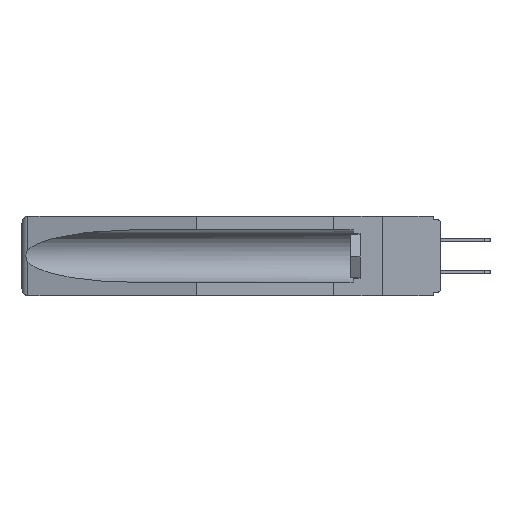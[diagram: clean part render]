
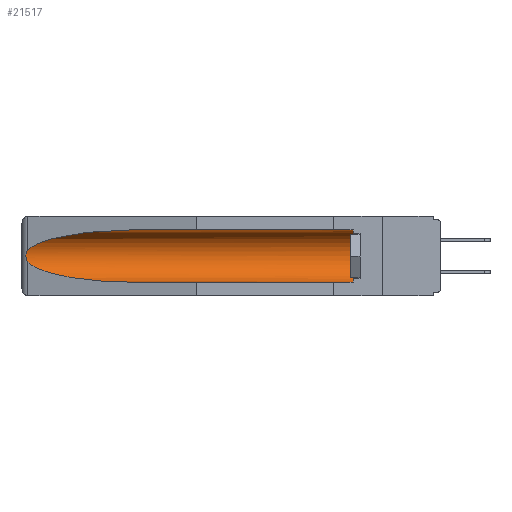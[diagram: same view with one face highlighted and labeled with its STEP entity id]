
A CAD part, left-side view. The second image highlights one B-rep face of the part: STEP entity #21517.
In plain terms, the highlighted cylindrical face has radius 2.857 mm (diameter 5.715 mm), a partial arc.
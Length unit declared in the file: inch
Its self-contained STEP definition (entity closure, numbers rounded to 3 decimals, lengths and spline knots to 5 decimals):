
#152 = EDGE_CURVE ( 'NONE', #22144, #23970, #13756, .T. ) ;
#161 = CARTESIAN_POINT ( 'NONE',  ( 0.26537, 1.52718, -0.19328 ) ) ;
#1623 = VECTOR ( 'NONE', #29195, 39.37008 ) ;
#1887 = VECTOR ( 'NONE', #17776, 39.37008 ) ;
#2953 = CARTESIAN_POINT ( 'NONE',  ( 0.155, 1.07973, -0.284 ) ) ;
#3125 = CARTESIAN_POINT ( 'NONE',  ( 0.26597, 1.52961, -0.15275 ) ) ;
#3984 = CARTESIAN_POINT ( 'NONE',  ( 0.26537, 1.52718, -0.14972 ) ) ;
#4189 =( BOUNDED_CURVE ( )  B_SPLINE_CURVE ( 3, ( #23513, #18738, #16533, #2953 ),
 .UNSPECIFIED., .F., .T. ) 
 B_SPLINE_CURVE_WITH_KNOTS ( ( 4, 4 ),
 ( 0.1948, 1.5708 ),
 .UNSPECIFIED. ) 
 CURVE ( )  GEOMETRIC_REPRESENTATION_ITEM ( )  RATIONAL_B_SPLINE_CURVE ( ( 1., 0.848, 0.848, 1. ) ) 
 REPRESENTATION_ITEM ( '' )  );
#6234 = ORIENTED_EDGE ( 'NONE', *, *, #152, .T. ) ;
#6364 = AXIS2_PLACEMENT_3D ( 'NONE', #8377, #15535, #26791 ) ;
#7174 = CARTESIAN_POINT ( 'NONE',  ( 0.155, 0.126, -0.284 ) ) ;
#7313 = DIRECTION ( 'NONE',  ( 0., -1., 0. ) ) ;
#8034 = CARTESIAN_POINT ( 'NONE',  ( 0.2673, 1.53269, -0.17917 ) ) ;
#8248 = ORIENTED_EDGE ( 'NONE', *, *, #8901, .T. ) ;
#8377 = CARTESIAN_POINT ( 'NONE',  ( 0.155, -0.30754, -0.1715 ) ) ;
#8474 = EDGE_CURVE ( 'NONE', #22722, #29050, #4189, .T. ) ;
#8792 = CARTESIAN_POINT ( 'NONE',  ( 0.21114, 1.30732, -0.059 ) ) ;
#8901 = EDGE_CURVE ( 'NONE', #23970, #8957, #28497, .T. ) ;
#8957 = VERTEX_POINT ( 'NONE', #24728 ) ;
#9082 = CARTESIAN_POINT ( 'NONE',  ( 0.155, -0.30754, -0.059 ) ) ;
#10154 = ORIENTED_EDGE ( 'NONE', *, *, #8474, .T. ) ;
#10318 = CARTESIAN_POINT ( 'NONE',  ( 0.2675, 1.53308, -0.17534 ) ) ;
#10955 = CARTESIAN_POINT ( 'NONE',  ( 0.155, -0.30754, -0.284 ) ) ;
#12690 = CARTESIAN_POINT ( 'NONE',  ( 0.26537, 1.52718, -0.19328 ) ) ;
#12919 = CIRCLE ( 'NONE', #18599, 0.1125 ) ;
#13147 = CARTESIAN_POINT ( 'NONE',  ( 0.25451, 1.48313, -0.09465 ) ) ;
#13756 = LINE ( 'NONE', #9082, #1623 ) ;
#13889 = EDGE_LOOP ( 'NONE', ( #8248, #21753, #10154, #23943, #27142, #6234 ) ) ;
#14043 = FACE_OUTER_BOUND ( 'NONE', #13889, .T. ) ;
#14354 = DIRECTION ( 'NONE',  ( 0., 0., 1. ) ) ;
#14788 = CARTESIAN_POINT ( 'NONE',  ( 0.26655, 1.53094, -0.18657 ) ) ;
#15535 = DIRECTION ( 'NONE',  ( 0., 1., 0. ) ) ;
#16533 = CARTESIAN_POINT ( 'NONE',  ( 0.21114, 1.30732, -0.284 ) ) ;
#17128 = EDGE_CURVE ( 'NONE', #8957, #22722, #17936, .T. ) ;
#17313 = CARTESIAN_POINT ( 'NONE',  ( 0.26654, 1.53092, -0.15636 ) ) ;
#17776 = DIRECTION ( 'NONE',  ( 0., 1., 0. ) ) ;
#17936 = B_SPLINE_CURVE_WITH_KNOTS ( 'NONE', 3,
 ( #27565, #3125, #17313, #19966, #26466, #10318, #8034, #14788, #24177, #12690 ),
 .UNSPECIFIED., .F., .F.,
 ( 4, 2, 2, 2, 4 ),
 ( 0., 0.00029, 0.00058, 0.00087, 0.00117 ),
 .UNSPECIFIED. ) ;
#18102 = VERTEX_POINT ( 'NONE', #7174 ) ;
#18599 = AXIS2_PLACEMENT_3D ( 'NONE', #28017, #7313, #14354 ) ;
#18738 = CARTESIAN_POINT ( 'NONE',  ( 0.25451, 1.48313, -0.24835 ) ) ;
#19966 = CARTESIAN_POINT ( 'NONE',  ( 0.2673, 1.5327, -0.16383 ) ) ;
#21163 = CYLINDRICAL_SURFACE ( 'NONE', #6364, 0.1125 ) ;
#21517 = ADVANCED_FACE ( 'NONE', ( #14043 ), #21163, .F. ) ;
#21753 = ORIENTED_EDGE ( 'NONE', *, *, #17128, .T. ) ;
#22144 = VERTEX_POINT ( 'NONE', #26959 ) ;
#22265 = EDGE_CURVE ( 'NONE', #18102, #22144, #12919, .T. ) ;
#22333 = CARTESIAN_POINT ( 'NONE',  ( 0.155, 1.07973, -0.059 ) ) ;
#22722 = VERTEX_POINT ( 'NONE', #161 ) ;
#23412 = CARTESIAN_POINT ( 'NONE',  ( 0.155, 1.07973, -0.059 ) ) ;
#23513 = CARTESIAN_POINT ( 'NONE',  ( 0.26537, 1.52718, -0.19328 ) ) ;
#23686 = CARTESIAN_POINT ( 'NONE',  ( 0.155, 1.07973, -0.284 ) ) ;
#23943 = ORIENTED_EDGE ( 'NONE', *, *, #26262, .F. ) ;
#23970 = VERTEX_POINT ( 'NONE', #23412 ) ;
#24177 = CARTESIAN_POINT ( 'NONE',  ( 0.26597, 1.5296, -0.19026 ) ) ;
#24728 = CARTESIAN_POINT ( 'NONE',  ( 0.26537, 1.52718, -0.14972 ) ) ;
#26262 = EDGE_CURVE ( 'NONE', #18102, #29050, #29359, .T. ) ;
#26466 = CARTESIAN_POINT ( 'NONE',  ( 0.2675, 1.53308, -0.16763 ) ) ;
#26791 = DIRECTION ( 'NONE',  ( 0., 0., 1. ) ) ;
#26959 = CARTESIAN_POINT ( 'NONE',  ( 0.155, 0.126, -0.059 ) ) ;
#27142 = ORIENTED_EDGE ( 'NONE', *, *, #22265, .T. ) ;
#27565 = CARTESIAN_POINT ( 'NONE',  ( 0.26537, 1.52718, -0.14972 ) ) ;
#28017 = CARTESIAN_POINT ( 'NONE',  ( 0.155, 0.126, -0.1715 ) ) ;
#28497 =( BOUNDED_CURVE ( )  B_SPLINE_CURVE ( 3, ( #22333, #8792, #13147, #3984 ),
 .UNSPECIFIED., .F., .F. ) 
 B_SPLINE_CURVE_WITH_KNOTS ( ( 4, 4 ),
 ( 4.71239, 6.08839 ),
 .UNSPECIFIED. ) 
 CURVE ( )  GEOMETRIC_REPRESENTATION_ITEM ( )  RATIONAL_B_SPLINE_CURVE ( ( 1., 0.848, 0.848, 1. ) ) 
 REPRESENTATION_ITEM ( '' )  );
#29050 = VERTEX_POINT ( 'NONE', #23686 ) ;
#29195 = DIRECTION ( 'NONE',  ( 0., 1., 0. ) ) ;
#29359 = LINE ( 'NONE', #10955, #1887 ) ;
